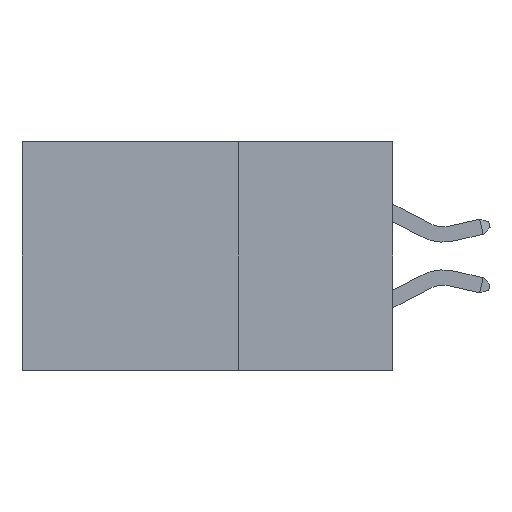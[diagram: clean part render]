
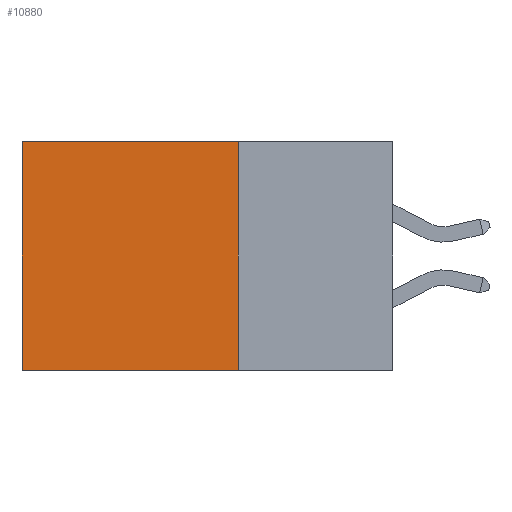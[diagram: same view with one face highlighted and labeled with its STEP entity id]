
A CAD part, left-side view. The second image highlights one B-rep face of the part: STEP entity #10880.
In plain terms, the highlighted planar face has unit normal (-1, 0, 0).
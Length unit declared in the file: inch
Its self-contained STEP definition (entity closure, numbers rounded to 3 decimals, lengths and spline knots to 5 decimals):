
#864 = LINE ( 'NONE', #16970, #23766 ) ;
#1108 = LINE ( 'NONE', #11451, #4226 ) ;
#1688 = EDGE_CURVE ( 'NONE', #18459, #7550, #17597, .T. ) ;
#2878 = CARTESIAN_POINT ( 'NONE',  ( 0.2875, 0.25, 0. ) ) ;
#4226 = VECTOR ( 'NONE', #11576, 39.37008 ) ;
#4468 = AXIS2_PLACEMENT_3D ( 'NONE', #19400, #13541, #21416 ) ;
#7442 = CARTESIAN_POINT ( 'NONE',  ( 0.2875, 0.25, 0. ) ) ;
#7483 = DIRECTION ( 'NONE',  ( 0., 0., -1. ) ) ;
#7498 = FACE_OUTER_BOUND ( 'NONE', #24589, .T. ) ;
#7550 = VERTEX_POINT ( 'NONE', #18219 ) ;
#8402 = ORIENTED_EDGE ( 'NONE', *, *, #13059, .T. ) ;
#9305 = CARTESIAN_POINT ( 'NONE',  ( 0.2875, 0.6, -0.37 ) ) ;
#10128 = VERTEX_POINT ( 'NONE', #24408 ) ;
#10880 = ADVANCED_FACE ( 'NONE', ( #7498 ), #25576, .F. ) ;
#11451 = CARTESIAN_POINT ( 'NONE',  ( 0.2875, 0.25, -0.37 ) ) ;
#11466 = DIRECTION ( 'NONE',  ( 0., 0., -1. ) ) ;
#11576 = DIRECTION ( 'NONE',  ( 0., 1., 0. ) ) ;
#11774 = CARTESIAN_POINT ( 'NONE',  ( 0.2875, 0.25, 0. ) ) ;
#13059 = EDGE_CURVE ( 'NONE', #7550, #21331, #864, .T. ) ;
#13541 = DIRECTION ( 'NONE',  ( 1., 0., 0. ) ) ;
#13787 = LINE ( 'NONE', #11774, #24007 ) ;
#15247 = DIRECTION ( 'NONE',  ( 0., 1., 0. ) ) ;
#16970 = CARTESIAN_POINT ( 'NONE',  ( 0.2875, 0.6, 0. ) ) ;
#17597 = LINE ( 'NONE', #7442, #19977 ) ;
#18219 = CARTESIAN_POINT ( 'NONE',  ( 0.2875, 0.6, 0. ) ) ;
#18459 = VERTEX_POINT ( 'NONE', #2878 ) ;
#19080 = EDGE_CURVE ( 'NONE', #18459, #10128, #13787, .T. ) ;
#19400 = CARTESIAN_POINT ( 'NONE',  ( 0.2875, 0.25, 0. ) ) ;
#19977 = VECTOR ( 'NONE', #15247, 39.37008 ) ;
#20879 = ORIENTED_EDGE ( 'NONE', *, *, #22633, .F. ) ;
#21331 = VERTEX_POINT ( 'NONE', #9305 ) ;
#21416 = DIRECTION ( 'NONE',  ( 0., 0., -1. ) ) ;
#22633 = EDGE_CURVE ( 'NONE', #10128, #21331, #1108, .T. ) ;
#23157 = ORIENTED_EDGE ( 'NONE', *, *, #1688, .T. ) ;
#23300 = ORIENTED_EDGE ( 'NONE', *, *, #19080, .F. ) ;
#23766 = VECTOR ( 'NONE', #11466, 39.37008 ) ;
#24007 = VECTOR ( 'NONE', #7483, 39.37008 ) ;
#24408 = CARTESIAN_POINT ( 'NONE',  ( 0.2875, 0.25, -0.37 ) ) ;
#24589 = EDGE_LOOP ( 'NONE', ( #8402, #20879, #23300, #23157 ) ) ;
#25576 = PLANE ( 'NONE',  #4468 ) ;
